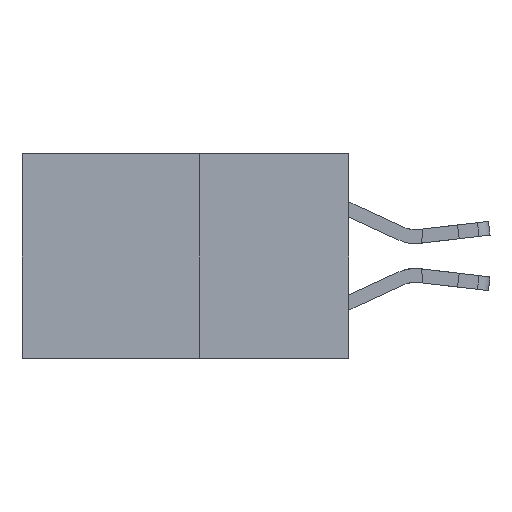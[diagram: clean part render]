
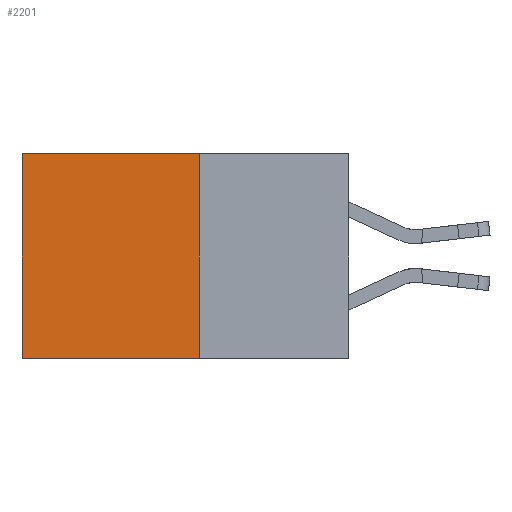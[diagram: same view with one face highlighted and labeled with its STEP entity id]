
A CAD part, left-side view. The second image highlights one B-rep face of the part: STEP entity #2201.
In plain terms, the highlighted planar face has unit normal (-1, 0, 0).
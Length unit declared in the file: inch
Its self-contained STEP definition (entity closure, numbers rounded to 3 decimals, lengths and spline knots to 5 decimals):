
#9 = VERTEX_POINT ( 'NONE', #12563 ) ;
#1222 = VECTOR ( 'NONE', #13505, 39.37008 ) ;
#1751 = VECTOR ( 'NONE', #19531, 39.37008 ) ;
#2201 = ADVANCED_FACE ( 'NONE', ( #11403 ), #9893, .F. ) ;
#3883 = CARTESIAN_POINT ( 'NONE',  ( 0.277, 0.27, -0.37 ) ) ;
#4474 = CARTESIAN_POINT ( 'NONE',  ( 0.277, 0.59, -0.37 ) ) ;
#6244 = LINE ( 'NONE', #4474, #1751 ) ;
#8777 = LINE ( 'NONE', #25698, #25128 ) ;
#9660 = VERTEX_POINT ( 'NONE', #12137 ) ;
#9893 = PLANE ( 'NONE',  #16366 ) ;
#10434 = DIRECTION ( 'NONE',  ( 0., 0., -1. ) ) ;
#11316 = CARTESIAN_POINT ( 'NONE',  ( 0.277, 0.27, 0. ) ) ;
#11403 = FACE_OUTER_BOUND ( 'NONE', #12653, .T. ) ;
#12136 = LINE ( 'NONE', #11316, #1222 ) ;
#12137 = CARTESIAN_POINT ( 'NONE',  ( 0.277, 0.27, -0.37 ) ) ;
#12563 = CARTESIAN_POINT ( 'NONE',  ( 0.277, 0.59, -0.37 ) ) ;
#12653 = EDGE_LOOP ( 'NONE', ( #24087, #23533, #13642, #21883 ) ) ;
#13505 = DIRECTION ( 'NONE',  ( 0., 1., 0. ) ) ;
#13642 = ORIENTED_EDGE ( 'NONE', *, *, #18057, .F. ) ;
#16366 = AXIS2_PLACEMENT_3D ( 'NONE', #25186, #22981, #25315 ) ;
#16468 = VERTEX_POINT ( 'NONE', #17641 ) ;
#16624 = LINE ( 'NONE', #3883, #27180 ) ;
#17641 = CARTESIAN_POINT ( 'NONE',  ( 0.277, 0.27, 0. ) ) ;
#18057 = EDGE_CURVE ( 'NONE', #16468, #9660, #16624, .T. ) ;
#19531 = DIRECTION ( 'NONE',  ( 0., 0., -1. ) ) ;
#20177 = EDGE_CURVE ( 'NONE', #22429, #9, #6244, .T. ) ;
#21883 = ORIENTED_EDGE ( 'NONE', *, *, #27361, .T. ) ;
#22429 = VERTEX_POINT ( 'NONE', #25513 ) ;
#22981 = DIRECTION ( 'NONE',  ( 1., 0., 0. ) ) ;
#23050 = DIRECTION ( 'NONE',  ( 0., 1., 0. ) ) ;
#23533 = ORIENTED_EDGE ( 'NONE', *, *, #27089, .F. ) ;
#24087 = ORIENTED_EDGE ( 'NONE', *, *, #20177, .T. ) ;
#25128 = VECTOR ( 'NONE', #23050, 39.37008 ) ;
#25186 = CARTESIAN_POINT ( 'NONE',  ( 0.277, 0.27, -0.37 ) ) ;
#25315 = DIRECTION ( 'NONE',  ( 0., 0., -1. ) ) ;
#25513 = CARTESIAN_POINT ( 'NONE',  ( 0.277, 0.59, 0. ) ) ;
#25698 = CARTESIAN_POINT ( 'NONE',  ( 0.277, 0.27, -0.37 ) ) ;
#27089 = EDGE_CURVE ( 'NONE', #9660, #9, #8777, .T. ) ;
#27180 = VECTOR ( 'NONE', #10434, 39.37008 ) ;
#27361 = EDGE_CURVE ( 'NONE', #16468, #22429, #12136, .T. ) ;
